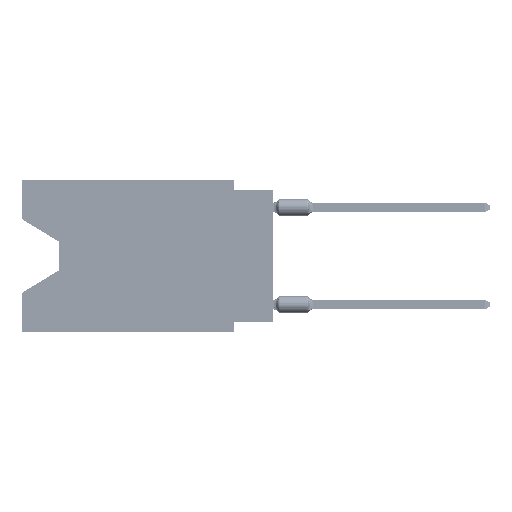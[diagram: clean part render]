
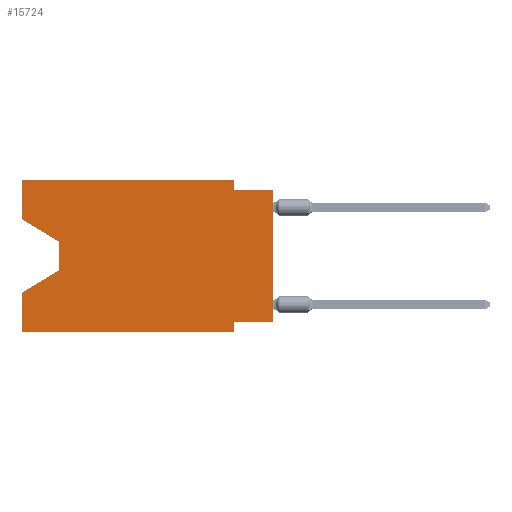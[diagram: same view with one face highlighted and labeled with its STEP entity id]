
A CAD part, left-side view. The second image highlights one B-rep face of the part: STEP entity #15724.
In plain terms, the highlighted planar face has unit normal (-1, 0, 0).
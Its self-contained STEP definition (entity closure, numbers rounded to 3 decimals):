
#348 = CARTESIAN_POINT ( 'NONE',  ( 0., 16.383, -9.906 ) ) ;
#1110 = CARTESIAN_POINT ( 'NONE',  ( 0., 16.383, -7.36 ) ) ;
#2153 = LINE ( 'NONE', #6802, #15849 ) ;
#5609 = CARTESIAN_POINT ( 'NONE',  ( 0., 16.383, 0. ) ) ;
#5742 = LINE ( 'NONE', #12145, #51676 ) ;
#6802 = CARTESIAN_POINT ( 'NONE',  ( 0., 16.383, 0. ) ) ;
#7136 = DIRECTION ( 'NONE',  ( 0., 1., 0. ) ) ;
#7166 = CARTESIAN_POINT ( 'NONE',  ( 0., 16.383, 0. ) ) ;
#8226 = DIRECTION ( 'NONE',  ( 0., 0., -1. ) ) ;
#8333 = EDGE_CURVE ( 'NONE', #65538, #31016, #37512, .T. ) ;
#8873 = VECTOR ( 'NONE', #32965, 1000. ) ;
#9770 = CARTESIAN_POINT ( 'NONE',  ( 0., 2.54, -9.271 ) ) ;
#10564 = CARTESIAN_POINT ( 'NONE',  ( 0., 2.54, 0. ) ) ;
#11234 = EDGE_CURVE ( 'NONE', #42863, #56161, #30017, .T. ) ;
#11239 = CARTESIAN_POINT ( 'NONE',  ( 0., 2.54, 0. ) ) ;
#12145 = CARTESIAN_POINT ( 'NONE',  ( 0., 0., -0.635 ) ) ;
#12189 = CARTESIAN_POINT ( 'NONE',  ( 0., 2.54, -0.635 ) ) ;
#12758 = ORIENTED_EDGE ( 'NONE', *, *, #21077, .T. ) ;
#13067 = DIRECTION ( 'NONE',  ( 0., -1., 0. ) ) ;
#13641 = DIRECTION ( 'NONE',  ( 0., 0.855, -0.519 ) ) ;
#14123 = DIRECTION ( 'NONE',  ( 0., 0., -1. ) ) ;
#14127 = ORIENTED_EDGE ( 'NONE', *, *, #8333, .T. ) ;
#14182 = ORIENTED_EDGE ( 'NONE', *, *, #68919, .F. ) ;
#15724 = ADVANCED_FACE ( 'NONE', ( #34250 ), #18918, .F. ) ;
#15849 = VECTOR ( 'NONE', #19501, 1000. ) ;
#16822 = CARTESIAN_POINT ( 'NONE',  ( 0., 0., 0. ) ) ;
#17401 = VERTEX_POINT ( 'NONE', #62313 ) ;
#17998 = CARTESIAN_POINT ( 'NONE',  ( 0., 13.97, -4.013 ) ) ;
#18403 = ORIENTED_EDGE ( 'NONE', *, *, #70107, .F. ) ;
#18576 = DIRECTION ( 'NONE',  ( 1., 0., 0. ) ) ;
#18918 = PLANE ( 'NONE',  #64365 ) ;
#19426 = EDGE_CURVE ( 'NONE', #31016, #42863, #28081, .T. ) ;
#19501 = DIRECTION ( 'NONE',  ( 0., -1., 0. ) ) ;
#19678 = CARTESIAN_POINT ( 'NONE',  ( 0., 13.97, -5.893 ) ) ;
#20529 = LINE ( 'NONE', #31222, #52054 ) ;
#21077 = EDGE_CURVE ( 'NONE', #53308, #41978, #61863, .T. ) ;
#21328 = CARTESIAN_POINT ( 'NONE',  ( 0., 0., -9.271 ) ) ;
#21833 = VECTOR ( 'NONE', #13067, 1000. ) ;
#26793 = EDGE_CURVE ( 'NONE', #60377, #17401, #5742, .T. ) ;
#26802 = LINE ( 'NONE', #16822, #31756 ) ;
#27015 = VECTOR ( 'NONE', #43003, 1000. ) ;
#27830 = DIRECTION ( 'NONE',  ( 0., 0., 1. ) ) ;
#27957 = VECTOR ( 'NONE', #27830, 1000. ) ;
#28068 = EDGE_CURVE ( 'NONE', #65538, #37496, #66672, .T. ) ;
#28081 = LINE ( 'NONE', #28800, #43264 ) ;
#28800 = CARTESIAN_POINT ( 'NONE',  ( 0., 13.97, -4.013 ) ) ;
#29992 = VECTOR ( 'NONE', #13641, 1000. ) ;
#30017 = LINE ( 'NONE', #19678, #29992 ) ;
#31016 = VERTEX_POINT ( 'NONE', #17998 ) ;
#31131 = ORIENTED_EDGE ( 'NONE', *, *, #58299, .F. ) ;
#31222 = CARTESIAN_POINT ( 'NONE',  ( 0., 0., -9.271 ) ) ;
#31756 = VECTOR ( 'NONE', #54924, 1000. ) ;
#32965 = DIRECTION ( 'NONE',  ( 0., 0., -1. ) ) ;
#33363 = ORIENTED_EDGE ( 'NONE', *, *, #57145, .T. ) ;
#34250 = FACE_OUTER_BOUND ( 'NONE', #46827, .T. ) ;
#35633 = VERTEX_POINT ( 'NONE', #21328 ) ;
#37156 = CARTESIAN_POINT ( 'NONE',  ( 0., 16.383, -2.546 ) ) ;
#37496 = VERTEX_POINT ( 'NONE', #43148 ) ;
#37512 = LINE ( 'NONE', #37156, #59329 ) ;
#41169 = LINE ( 'NONE', #62921, #42113 ) ;
#41978 = VERTEX_POINT ( 'NONE', #44729 ) ;
#42113 = VECTOR ( 'NONE', #14123, 1000. ) ;
#42863 = VERTEX_POINT ( 'NONE', #69332 ) ;
#43003 = DIRECTION ( 'NONE',  ( 0., 0., 1. ) ) ;
#43148 = CARTESIAN_POINT ( 'NONE',  ( 0., 16.383, 0. ) ) ;
#43264 = VECTOR ( 'NONE', #50507, 1000. ) ;
#43437 = ORIENTED_EDGE ( 'NONE', *, *, #26793, .F. ) ;
#44334 = VERTEX_POINT ( 'NONE', #10564 ) ;
#44729 = CARTESIAN_POINT ( 'NONE',  ( 0., 2.54, -9.906 ) ) ;
#44894 = DIRECTION ( 'NONE',  ( 0., -1., 0. ) ) ;
#45504 = CARTESIAN_POINT ( 'NONE',  ( 0., 16.383, -2.546 ) ) ;
#45864 = VERTEX_POINT ( 'NONE', #9770 ) ;
#46827 = EDGE_LOOP ( 'NONE', ( #14127, #51972, #57759, #18403, #12758, #31131, #14182, #33363, #43437, #46894, #54375, #47595 ) ) ;
#46894 = ORIENTED_EDGE ( 'NONE', *, *, #67954, .F. ) ;
#47595 = ORIENTED_EDGE ( 'NONE', *, *, #28068, .F. ) ;
#50507 = DIRECTION ( 'NONE',  ( 0., 0., -1. ) ) ;
#50740 = LINE ( 'NONE', #11239, #8873 ) ;
#51676 = VECTOR ( 'NONE', #44894, 1000. ) ;
#51824 = CARTESIAN_POINT ( 'NONE',  ( 0., 16.383, -9.906 ) ) ;
#51972 = ORIENTED_EDGE ( 'NONE', *, *, #19426, .T. ) ;
#52054 = VECTOR ( 'NONE', #7136, 1000. ) ;
#53308 = VERTEX_POINT ( 'NONE', #51824 ) ;
#54375 = ORIENTED_EDGE ( 'NONE', *, *, #54821, .F. ) ;
#54821 = EDGE_CURVE ( 'NONE', #37496, #44334, #2153, .T. ) ;
#54924 = DIRECTION ( 'NONE',  ( 0., 0., 1. ) ) ;
#55538 = DIRECTION ( 'NONE',  ( 0., -0.855, -0.519 ) ) ;
#56161 = VERTEX_POINT ( 'NONE', #1110 ) ;
#57145 = EDGE_CURVE ( 'NONE', #35633, #17401, #26802, .T. ) ;
#57759 = ORIENTED_EDGE ( 'NONE', *, *, #11234, .T. ) ;
#58299 = EDGE_CURVE ( 'NONE', #45864, #41978, #41169, .T. ) ;
#59329 = VECTOR ( 'NONE', #55538, 1000. ) ;
#60377 = VERTEX_POINT ( 'NONE', #12189 ) ;
#61863 = LINE ( 'NONE', #348, #21833 ) ;
#62313 = CARTESIAN_POINT ( 'NONE',  ( 0., 0., -0.635 ) ) ;
#62921 = CARTESIAN_POINT ( 'NONE',  ( 0., 2.54, -9.906 ) ) ;
#64365 = AXIS2_PLACEMENT_3D ( 'NONE', #67030, #18576, #8226 ) ;
#64414 = LINE ( 'NONE', #5609, #27015 ) ;
#65538 = VERTEX_POINT ( 'NONE', #45504 ) ;
#66672 = LINE ( 'NONE', #7166, #27957 ) ;
#67030 = CARTESIAN_POINT ( 'NONE',  ( 0., 16.383, 0. ) ) ;
#67954 = EDGE_CURVE ( 'NONE', #44334, #60377, #50740, .T. ) ;
#68919 = EDGE_CURVE ( 'NONE', #35633, #45864, #20529, .T. ) ;
#69332 = CARTESIAN_POINT ( 'NONE',  ( 0., 13.97, -5.893 ) ) ;
#70107 = EDGE_CURVE ( 'NONE', #53308, #56161, #64414, .T. ) ;
